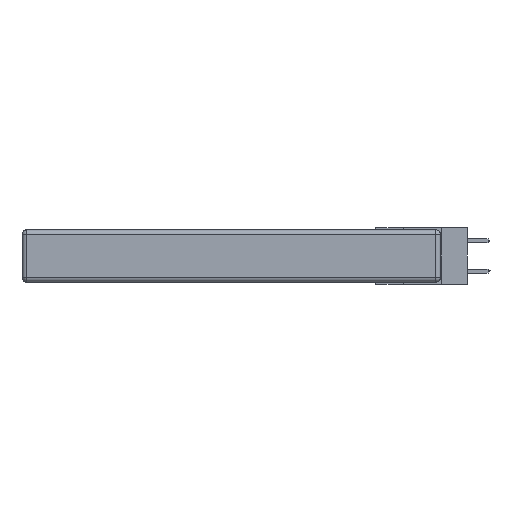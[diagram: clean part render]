
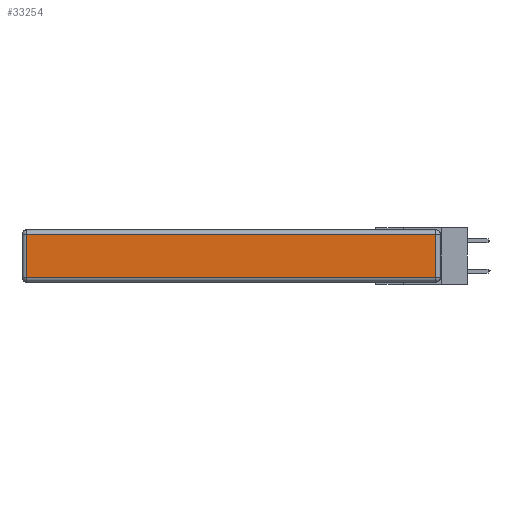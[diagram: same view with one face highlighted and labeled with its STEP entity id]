
A CAD part, left-side view. The second image highlights one B-rep face of the part: STEP entity #33254.
In plain terms, the highlighted planar face has unit normal (-1, 0, 0).
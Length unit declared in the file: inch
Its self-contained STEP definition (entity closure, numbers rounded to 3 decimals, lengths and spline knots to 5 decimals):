
#416 = DIRECTION ( 'NONE',  ( 0., -1., 0. ) ) ;
#2310 = VERTEX_POINT ( 'NONE', #5263 ) ;
#3315 = CARTESIAN_POINT ( 'NONE',  ( 0., 0., -0.343 ) ) ;
#4465 = VECTOR ( 'NONE', #416, 39.37008 ) ;
#4846 = ORIENTED_EDGE ( 'NONE', *, *, #5940, .T. ) ;
#5263 = CARTESIAN_POINT ( 'NONE',  ( 0., 0.03, -0.03 ) ) ;
#5603 = EDGE_CURVE ( 'NONE', #10459, #27226, #11691, .T. ) ;
#5838 = CARTESIAN_POINT ( 'NONE',  ( 0., 0., -0.313 ) ) ;
#5940 = EDGE_CURVE ( 'NONE', #2310, #26588, #21122, .T. ) ;
#7713 = CARTESIAN_POINT ( 'NONE',  ( 0., 2.72, -0.03 ) ) ;
#8888 = CARTESIAN_POINT ( 'NONE',  ( 0., 2.72, -0.313 ) ) ;
#10459 = VERTEX_POINT ( 'NONE', #8888 ) ;
#11047 = CARTESIAN_POINT ( 'NONE',  ( 0., 0.03, -0.313 ) ) ;
#11691 = LINE ( 'NONE', #5838, #4465 ) ;
#12803 = EDGE_CURVE ( 'NONE', #26588, #10459, #21530, .T. ) ;
#14191 = PLANE ( 'NONE',  #15425 ) ;
#15425 = AXIS2_PLACEMENT_3D ( 'NONE', #3315, #30700, #33361 ) ;
#15957 = CARTESIAN_POINT ( 'NONE',  ( 0., 0.03, -0.343 ) ) ;
#16403 = DIRECTION ( 'NONE',  ( 0., 0., -1. ) ) ;
#18143 = DIRECTION ( 'NONE',  ( 0., 1., 0. ) ) ;
#19570 = ORIENTED_EDGE ( 'NONE', *, *, #12803, .T. ) ;
#20451 = EDGE_LOOP ( 'NONE', ( #35215, #34348, #4846, #19570 ) ) ;
#21122 = LINE ( 'NONE', #23286, #26251 ) ;
#21386 = DIRECTION ( 'NONE',  ( 0., 0., 1. ) ) ;
#21530 = LINE ( 'NONE', #24898, #25794 ) ;
#23286 = CARTESIAN_POINT ( 'NONE',  ( 0., 2.75, -0.03 ) ) ;
#24898 = CARTESIAN_POINT ( 'NONE',  ( 0., 2.72, -0.343 ) ) ;
#25794 = VECTOR ( 'NONE', #16403, 39.37008 ) ;
#26251 = VECTOR ( 'NONE', #18143, 39.37008 ) ;
#26588 = VERTEX_POINT ( 'NONE', #7713 ) ;
#27226 = VERTEX_POINT ( 'NONE', #11047 ) ;
#29197 = EDGE_CURVE ( 'NONE', #27226, #2310, #33546, .T. ) ;
#30097 = VECTOR ( 'NONE', #21386, 39.37008 ) ;
#30700 = DIRECTION ( 'NONE',  ( -1., 0., 0. ) ) ;
#32680 = FACE_OUTER_BOUND ( 'NONE', #20451, .T. ) ;
#33254 = ADVANCED_FACE ( 'NONE', ( #32680 ), #14191, .T. ) ;
#33361 = DIRECTION ( 'NONE',  ( 0., 0., 1. ) ) ;
#33546 = LINE ( 'NONE', #15957, #30097 ) ;
#34348 = ORIENTED_EDGE ( 'NONE', *, *, #29197, .T. ) ;
#35215 = ORIENTED_EDGE ( 'NONE', *, *, #5603, .T. ) ;
